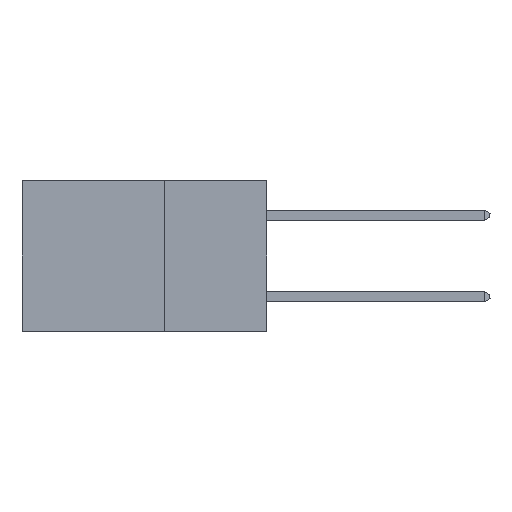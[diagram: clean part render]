
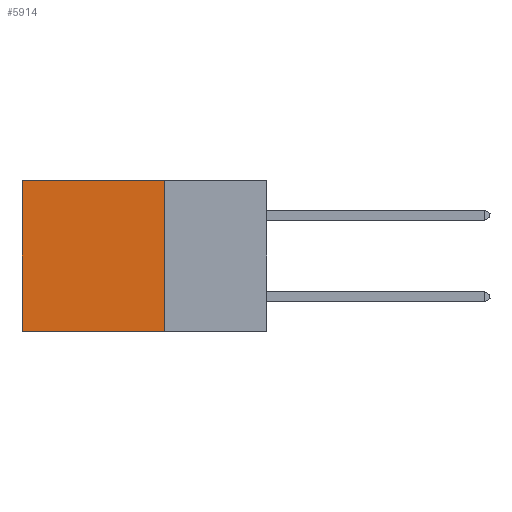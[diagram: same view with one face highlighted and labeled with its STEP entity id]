
A CAD part, left-side view. The second image highlights one B-rep face of the part: STEP entity #5914.
In plain terms, the highlighted planar face has unit normal (-1, 0, 0).
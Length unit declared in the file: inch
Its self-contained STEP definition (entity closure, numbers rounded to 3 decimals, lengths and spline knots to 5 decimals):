
#833 = DIRECTION ( 'NONE',  ( 0., 0., -1. ) ) ;
#1054 = VERTEX_POINT ( 'NONE', #24617 ) ;
#1308 = ORIENTED_EDGE ( 'NONE', *, *, #1873, .T. ) ;
#1545 = ORIENTED_EDGE ( 'NONE', *, *, #23094, .T. ) ;
#1873 = EDGE_CURVE ( 'NONE', #9408, #1054, #2986, .T. ) ;
#2301 = VERTEX_POINT ( 'NONE', #5035 ) ;
#2986 = LINE ( 'NONE', #22870, #16775 ) ;
#3372 = EDGE_CURVE ( 'NONE', #16358, #1054, #27965, .T. ) ;
#3795 = VECTOR ( 'NONE', #20190, 39.37008 ) ;
#4366 = FACE_OUTER_BOUND ( 'NONE', #14550, .T. ) ;
#4850 = CARTESIAN_POINT ( 'NONE',  ( 0.2875, 0.25, -0.37 ) ) ;
#5035 = CARTESIAN_POINT ( 'NONE',  ( 0.2875, 0.25, 0. ) ) ;
#5914 = ADVANCED_FACE ( 'NONE', ( #4366 ), #28665, .F. ) ;
#8703 = CARTESIAN_POINT ( 'NONE',  ( 0.2875, 0.25, -0.37 ) ) ;
#9408 = VERTEX_POINT ( 'NONE', #13566 ) ;
#11361 = LINE ( 'NONE', #15700, #16958 ) ;
#11818 = CARTESIAN_POINT ( 'NONE',  ( 0.2875, 0.25, 0. ) ) ;
#13337 = ORIENTED_EDGE ( 'NONE', *, *, #19724, .F. ) ;
#13566 = CARTESIAN_POINT ( 'NONE',  ( 0.2875, 0.6, 0. ) ) ;
#14550 = EDGE_LOOP ( 'NONE', ( #1308, #19447, #13337, #1545 ) ) ;
#15700 = CARTESIAN_POINT ( 'NONE',  ( 0.2875, 0.25, 0. ) ) ;
#16358 = VERTEX_POINT ( 'NONE', #4850 ) ;
#16568 = AXIS2_PLACEMENT_3D ( 'NONE', #11818, #31081, #16696 ) ;
#16696 = DIRECTION ( 'NONE',  ( 0., 0., -1. ) ) ;
#16775 = VECTOR ( 'NONE', #833, 39.37008 ) ;
#16958 = VECTOR ( 'NONE', #18115, 39.37008 ) ;
#18115 = DIRECTION ( 'NONE',  ( 0., 0., -1. ) ) ;
#19447 = ORIENTED_EDGE ( 'NONE', *, *, #3372, .F. ) ;
#19724 = EDGE_CURVE ( 'NONE', #2301, #16358, #11361, .T. ) ;
#20190 = DIRECTION ( 'NONE',  ( 0., 1., 0. ) ) ;
#20693 = DIRECTION ( 'NONE',  ( 0., 1., 0. ) ) ;
#21548 = VECTOR ( 'NONE', #20693, 39.37008 ) ;
#22870 = CARTESIAN_POINT ( 'NONE',  ( 0.2875, 0.6, 0. ) ) ;
#23094 = EDGE_CURVE ( 'NONE', #2301, #9408, #30324, .T. ) ;
#24617 = CARTESIAN_POINT ( 'NONE',  ( 0.2875, 0.6, -0.37 ) ) ;
#27340 = CARTESIAN_POINT ( 'NONE',  ( 0.2875, 0.25, 0. ) ) ;
#27965 = LINE ( 'NONE', #8703, #21548 ) ;
#28665 = PLANE ( 'NONE',  #16568 ) ;
#30324 = LINE ( 'NONE', #27340, #3795 ) ;
#31081 = DIRECTION ( 'NONE',  ( 1., 0., 0. ) ) ;
